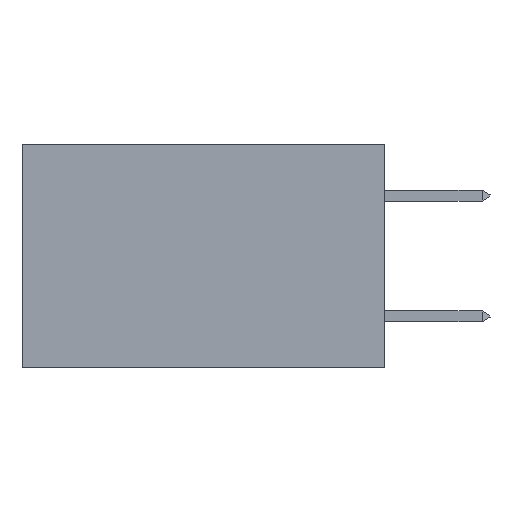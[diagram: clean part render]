
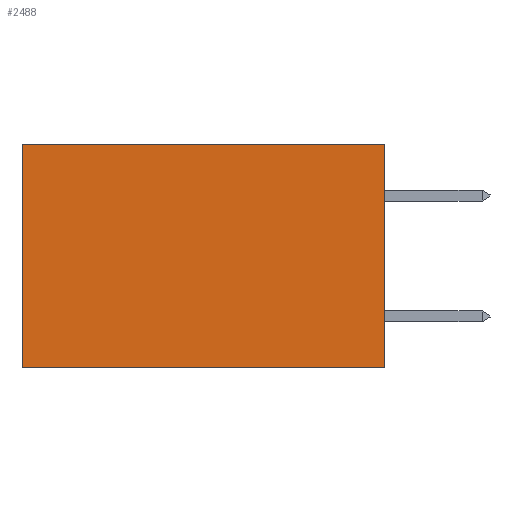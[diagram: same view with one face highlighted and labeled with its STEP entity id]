
A CAD part, left-side view. The second image highlights one B-rep face of the part: STEP entity #2488.
In plain terms, the highlighted planar face has unit normal (-1, 0, 0).
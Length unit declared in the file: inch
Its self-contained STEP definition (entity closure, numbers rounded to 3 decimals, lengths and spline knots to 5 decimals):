
#97 = LINE ( 'NONE', #1267, #12496 ) ;
#118 = EDGE_CURVE ( 'NONE', #16955, #4729, #4932, .T. ) ;
#317 = VERTEX_POINT ( 'NONE', #13588 ) ;
#687 = DIRECTION ( 'NONE',  ( 0., 0., -1. ) ) ;
#1267 = CARTESIAN_POINT ( 'NONE',  ( 0.2875, 0., -0.37 ) ) ;
#1973 = VECTOR ( 'NONE', #10943, 39.37008 ) ;
#2179 = AXIS2_PLACEMENT_3D ( 'NONE', #3451, #20402, #6757 ) ;
#2488 = ADVANCED_FACE ( 'NONE', ( #6885 ), #17336, .F. ) ;
#3451 = CARTESIAN_POINT ( 'NONE',  ( 0.2875, 0., 0. ) ) ;
#4729 = VERTEX_POINT ( 'NONE', #5643 ) ;
#4932 = LINE ( 'NONE', #16066, #8768 ) ;
#4956 = EDGE_LOOP ( 'NONE', ( #14196, #17053, #13945, #8560 ) ) ;
#5643 = CARTESIAN_POINT ( 'NONE',  ( 0.2875, 0., -0.37 ) ) ;
#6757 = DIRECTION ( 'NONE',  ( 0., 0., -1. ) ) ;
#6885 = FACE_OUTER_BOUND ( 'NONE', #4956, .T. ) ;
#7718 = CARTESIAN_POINT ( 'NONE',  ( 0.2875, 0.6, 0. ) ) ;
#8265 = DIRECTION ( 'NONE',  ( 0., 1., 0. ) ) ;
#8560 = ORIENTED_EDGE ( 'NONE', *, *, #9797, .T. ) ;
#8768 = VECTOR ( 'NONE', #687, 39.37008 ) ;
#8909 = LINE ( 'NONE', #19089, #16678 ) ;
#9797 = EDGE_CURVE ( 'NONE', #16955, #317, #8909, .T. ) ;
#10837 = EDGE_CURVE ( 'NONE', #317, #18405, #14233, .T. ) ;
#10943 = DIRECTION ( 'NONE',  ( 0., 0., -1. ) ) ;
#12496 = VECTOR ( 'NONE', #17097, 39.37008 ) ;
#12895 = CARTESIAN_POINT ( 'NONE',  ( 0.2875, 0., 0. ) ) ;
#13588 = CARTESIAN_POINT ( 'NONE',  ( 0.2875, 0.6, 0. ) ) ;
#13945 = ORIENTED_EDGE ( 'NONE', *, *, #118, .F. ) ;
#14196 = ORIENTED_EDGE ( 'NONE', *, *, #10837, .T. ) ;
#14233 = LINE ( 'NONE', #7718, #1973 ) ;
#16066 = CARTESIAN_POINT ( 'NONE',  ( 0.2875, 0., 0. ) ) ;
#16678 = VECTOR ( 'NONE', #8265, 39.37008 ) ;
#16955 = VERTEX_POINT ( 'NONE', #12895 ) ;
#17053 = ORIENTED_EDGE ( 'NONE', *, *, #17408, .F. ) ;
#17097 = DIRECTION ( 'NONE',  ( 0., 1., 0. ) ) ;
#17336 = PLANE ( 'NONE',  #2179 ) ;
#17408 = EDGE_CURVE ( 'NONE', #4729, #18405, #97, .T. ) ;
#18405 = VERTEX_POINT ( 'NONE', #19306 ) ;
#19089 = CARTESIAN_POINT ( 'NONE',  ( 0.2875, 0., 0. ) ) ;
#19306 = CARTESIAN_POINT ( 'NONE',  ( 0.2875, 0.6, -0.37 ) ) ;
#20402 = DIRECTION ( 'NONE',  ( 1., 0., 0. ) ) ;
